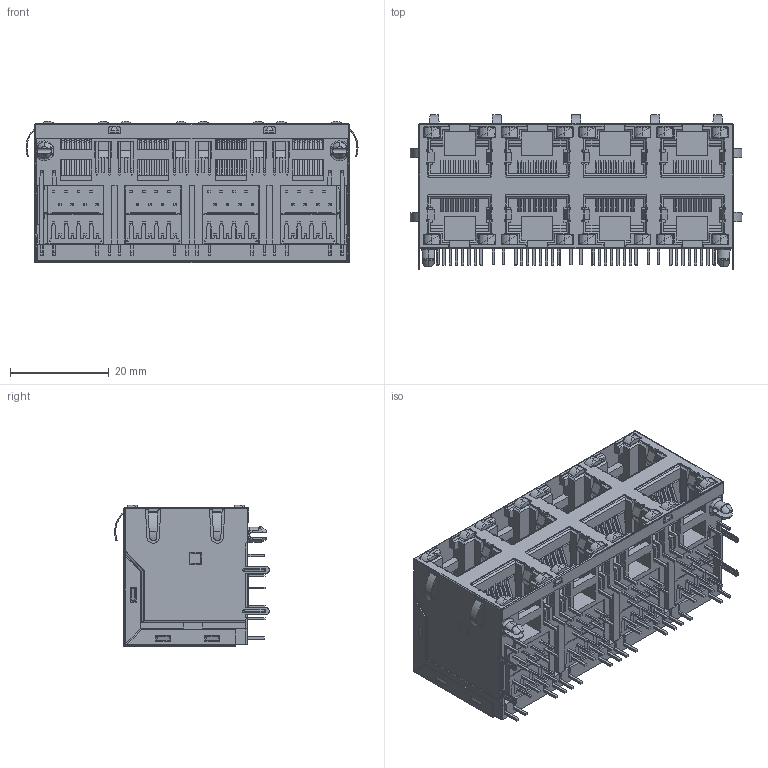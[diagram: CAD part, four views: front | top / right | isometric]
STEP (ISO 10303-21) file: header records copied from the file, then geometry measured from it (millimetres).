
FILE_DESCRIPTION (( 'STEP AP203' ), '1' );
FILE_NAME ('J96088892P85221.STEP', '2020-03-24T04:26:47', ( '' ), ( '' ), 'SwSTEP 2.0', 'SolidWorks 2016', '' );
FILE_SCHEMA (( 'CONFIG_CONTROL_DESIGN' ));
Length unit declared in the file: millimetre
Products named in the file (14): 96 Contacts Lower; 96 LED LH Upper_8-Red-Yellow; 96 Grounding_8 Ports; 96 Back Plate_8 Ports; 96 Contact Lock Upper; 96 LED RH Upper_5-Green-Yellow; J96088892P85221; 96 Shield_8 Ports LED - EMI; 96 LED LH Lower_8-Red-Yellow; 96 Contacts Upper; 96 Insulator Insert; 96 Contact Lock Lower; 96 Insulator_8 Ports; 96 LED RH Lower_5-Green-Yellow
Assembly tree (40 placements, depth 2):
  J96088892P85221
    96 Insulator_8 Ports
    96 LED LH Lower_8-Red-Yellow  x4
    96 LED RH Lower_5-Green-Yellow  x4
    96 Contacts Lower  x4
    96 Contact Lock Lower  x4
    96 Grounding_8 Ports
    96 Contacts Upper  x4
    96 Contact Lock Upper  x4
    96 Insulator Insert  x4
    96 LED LH Upper_8-Red-Yellow  x4
    96 LED RH Upper_5-Green-Yellow  x4
    96 Back Plate_8 Ports
    96 Shield_8 Ports LED - EMI
Bounding box: 67.35 x 31.38 x 28.68 mm (x, y, z)
Volume: 24148.5 mm3; surface area: 63596.2 mm2
Topology: 96 solids, 96 shells, 7836 faces, 21940 edges, 14070 vertices
Faces by surface type: plane 6105, cylinder 1420, bspline 297, cone 14
Entity records: 150132 total; most frequent: CARTESIAN_POINT 34861, ORIENTED_EDGE 25200, DIRECTION 21107, EDGE_CURVE 12600, VECTOR 10205, LINE 10205, VERTEX_POINT 8125, AXIS2_PLACEMENT_3D 5451
